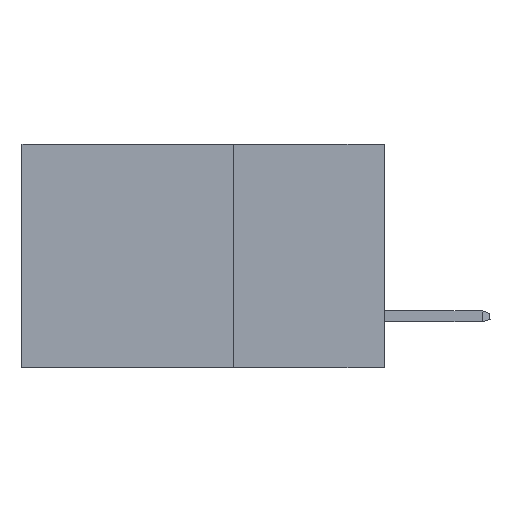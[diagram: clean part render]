
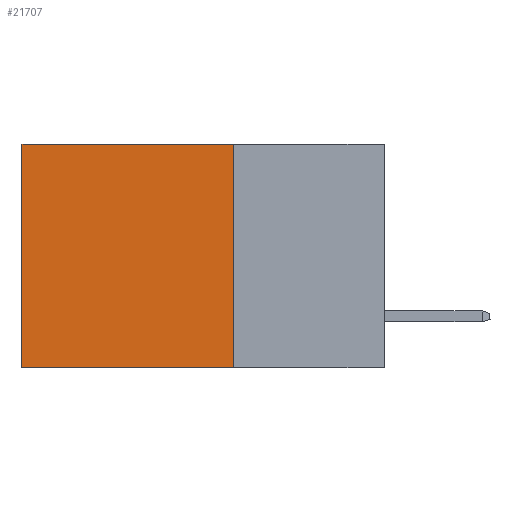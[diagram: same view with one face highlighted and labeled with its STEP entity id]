
A CAD part, left-side view. The second image highlights one B-rep face of the part: STEP entity #21707.
In plain terms, the highlighted planar face has unit normal (-1, 0, 0).
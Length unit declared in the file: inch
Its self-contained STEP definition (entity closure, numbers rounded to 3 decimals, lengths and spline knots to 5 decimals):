
#431 = CARTESIAN_POINT ( 'NONE',  ( 0.298, 0.6, -0.37 ) ) ;
#778 = DIRECTION ( 'NONE',  ( 0., 1., 0. ) ) ;
#997 = CARTESIAN_POINT ( 'NONE',  ( 0.298, 0.6, 0. ) ) ;
#1672 = VERTEX_POINT ( 'NONE', #3319 ) ;
#1922 = EDGE_LOOP ( 'NONE', ( #21646, #12572, #6209, #12360 ) ) ;
#2358 = VECTOR ( 'NONE', #16777, 39.37008 ) ;
#2570 = PLANE ( 'NONE',  #20936 ) ;
#3172 = EDGE_CURVE ( 'NONE', #17869, #1672, #15703, .T. ) ;
#3319 = CARTESIAN_POINT ( 'NONE',  ( 0.298, 0.6, 0. ) ) ;
#3710 = CARTESIAN_POINT ( 'NONE',  ( 0.298, 0.25, 0. ) ) ;
#3722 = DIRECTION ( 'NONE',  ( 0., 1., 0. ) ) ;
#4162 = DIRECTION ( 'NONE',  ( 1., 0., 0. ) ) ;
#5052 = VECTOR ( 'NONE', #12441, 39.37008 ) ;
#6209 = ORIENTED_EDGE ( 'NONE', *, *, #19472, .F. ) ;
#8324 = LINE ( 'NONE', #3710, #5052 ) ;
#9989 = LINE ( 'NONE', #14237, #16884 ) ;
#11028 = VECTOR ( 'NONE', #778, 39.37008 ) ;
#12360 = ORIENTED_EDGE ( 'NONE', *, *, #3172, .T. ) ;
#12441 = DIRECTION ( 'NONE',  ( 0., 0., -1. ) ) ;
#12572 = ORIENTED_EDGE ( 'NONE', *, *, #21608, .F. ) ;
#12716 = CARTESIAN_POINT ( 'NONE',  ( 0.298, 0.25, 0. ) ) ;
#14014 = CARTESIAN_POINT ( 'NONE',  ( 0.298, 0.25, 0. ) ) ;
#14237 = CARTESIAN_POINT ( 'NONE',  ( 0.298, 0.25, -0.37 ) ) ;
#14436 = LINE ( 'NONE', #997, #2358 ) ;
#14697 = CARTESIAN_POINT ( 'NONE',  ( 0.298, 0.25, 0. ) ) ;
#14701 = EDGE_CURVE ( 'NONE', #1672, #21695, #14436, .T. ) ;
#15450 = VERTEX_POINT ( 'NONE', #20857 ) ;
#15703 = LINE ( 'NONE', #12716, #11028 ) ;
#16777 = DIRECTION ( 'NONE',  ( 0., 0., -1. ) ) ;
#16884 = VECTOR ( 'NONE', #3722, 39.37008 ) ;
#17869 = VERTEX_POINT ( 'NONE', #14014 ) ;
#18351 = FACE_OUTER_BOUND ( 'NONE', #1922, .T. ) ;
#19472 = EDGE_CURVE ( 'NONE', #17869, #15450, #8324, .T. ) ;
#19858 = DIRECTION ( 'NONE',  ( 0., 0., -1. ) ) ;
#20857 = CARTESIAN_POINT ( 'NONE',  ( 0.298, 0.25, -0.37 ) ) ;
#20936 = AXIS2_PLACEMENT_3D ( 'NONE', #14697, #4162, #19858 ) ;
#21608 = EDGE_CURVE ( 'NONE', #15450, #21695, #9989, .T. ) ;
#21646 = ORIENTED_EDGE ( 'NONE', *, *, #14701, .T. ) ;
#21695 = VERTEX_POINT ( 'NONE', #431 ) ;
#21707 = ADVANCED_FACE ( 'NONE', ( #18351 ), #2570, .F. ) ;
